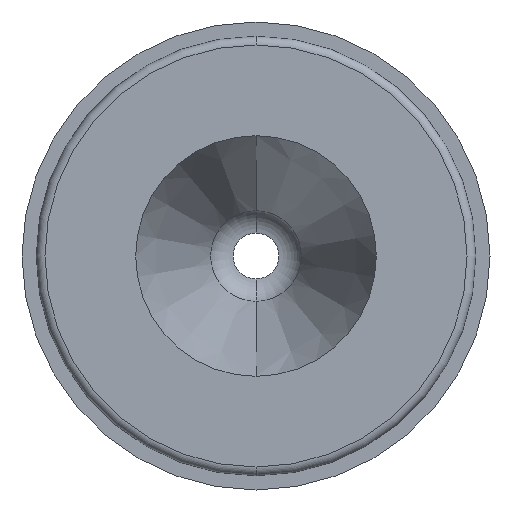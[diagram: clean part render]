
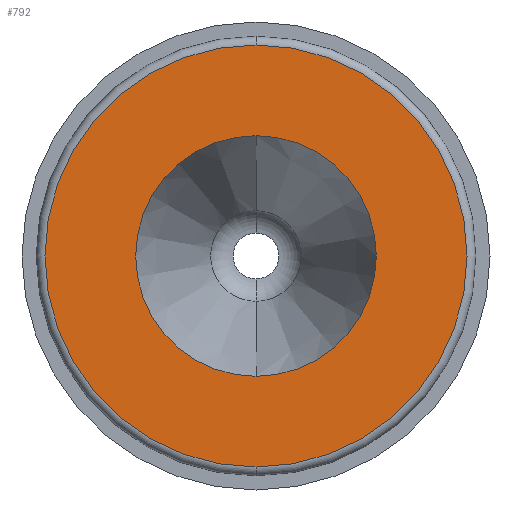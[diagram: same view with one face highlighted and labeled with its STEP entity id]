
A CAD part, front view. The second image highlights one B-rep face of the part: STEP entity #792.
In plain terms, the highlighted planar face has unit normal (0, -1, 0).
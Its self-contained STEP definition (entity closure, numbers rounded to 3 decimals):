
#5 = DIRECTION ( 'NONE',  ( 0., 0., -1. ) ) ;
#36 = CIRCLE ( 'NONE', #677, 22. ) ;
#38 = AXIS2_PLACEMENT_3D ( 'NONE', #222, #552, #290 ) ;
#46 = DIRECTION ( 'NONE',  ( 0., -1., 0. ) ) ;
#84 = CARTESIAN_POINT ( 'NONE',  ( 0., 0., 0. ) ) ;
#99 = ORIENTED_EDGE ( 'NONE', *, *, #608, .T. ) ;
#109 = EDGE_LOOP ( 'NONE', ( #186, #570 ) ) ;
#137 = CARTESIAN_POINT ( 'NONE',  ( 0., 0., -38.6 ) ) ;
#140 = DIRECTION ( 'NONE',  ( 0., -1., 0. ) ) ;
#179 = PLANE ( 'NONE',  #38 ) ;
#186 = ORIENTED_EDGE ( 'NONE', *, *, #187, .F. ) ;
#187 = EDGE_CURVE ( 'NONE', #439, #315, #36, .T. ) ;
#222 = CARTESIAN_POINT ( 'NONE',  ( -22., 0., 0. ) ) ;
#240 = CIRCLE ( 'NONE', #294, 22. ) ;
#273 = AXIS2_PLACEMENT_3D ( 'NONE', #544, #740, #5 ) ;
#278 = EDGE_CURVE ( 'NONE', #315, #439, #240, .T. ) ;
#290 = DIRECTION ( 'NONE',  ( 0., 0., 1. ) ) ;
#294 = AXIS2_PLACEMENT_3D ( 'NONE', #436, #443, #830 ) ;
#315 = VERTEX_POINT ( 'NONE', #833 ) ;
#322 = CARTESIAN_POINT ( 'NONE',  ( 0., 0., 0. ) ) ;
#345 = DIRECTION ( 'NONE',  ( 0., 0., -1. ) ) ;
#381 = FACE_OUTER_BOUND ( 'NONE', #476, .T. ) ;
#382 = ORIENTED_EDGE ( 'NONE', *, *, #764, .T. ) ;
#436 = CARTESIAN_POINT ( 'NONE',  ( 0., 0., 0. ) ) ;
#439 = VERTEX_POINT ( 'NONE', #576 ) ;
#443 = DIRECTION ( 'NONE',  ( 0., -1., 0. ) ) ;
#476 = EDGE_LOOP ( 'NONE', ( #99, #382 ) ) ;
#485 = AXIS2_PLACEMENT_3D ( 'NONE', #322, #46, #847 ) ;
#544 = CARTESIAN_POINT ( 'NONE',  ( 0., 0., 0. ) ) ;
#552 = DIRECTION ( 'NONE',  ( 0., 1., 0. ) ) ;
#570 = ORIENTED_EDGE ( 'NONE', *, *, #278, .F. ) ;
#576 = CARTESIAN_POINT ( 'NONE',  ( 0., 0., -22. ) ) ;
#608 = EDGE_CURVE ( 'NONE', #709, #781, #725, .T. ) ;
#617 = CARTESIAN_POINT ( 'NONE',  ( 0., 0., 38.6 ) ) ;
#677 = AXIS2_PLACEMENT_3D ( 'NONE', #84, #140, #345 ) ;
#700 = FACE_BOUND ( 'NONE', #109, .T. ) ;
#709 = VERTEX_POINT ( 'NONE', #137 ) ;
#725 = CIRCLE ( 'NONE', #485, 38.6 ) ;
#740 = DIRECTION ( 'NONE',  ( 0., -1., 0. ) ) ;
#764 = EDGE_CURVE ( 'NONE', #781, #709, #866, .T. ) ;
#781 = VERTEX_POINT ( 'NONE', #617 ) ;
#792 = ADVANCED_FACE ( 'NONE', ( #700, #381 ), #179, .F. ) ;
#830 = DIRECTION ( 'NONE',  ( 0., 0., -1. ) ) ;
#833 = CARTESIAN_POINT ( 'NONE',  ( 0., 0., 22. ) ) ;
#847 = DIRECTION ( 'NONE',  ( 0., 0., -1. ) ) ;
#866 = CIRCLE ( 'NONE', #273, 38.6 ) ;
